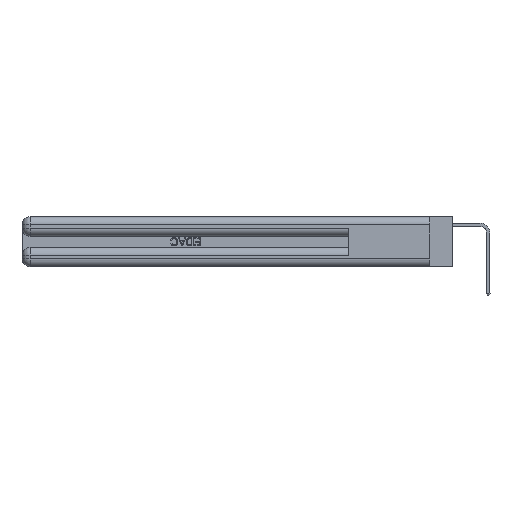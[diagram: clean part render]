
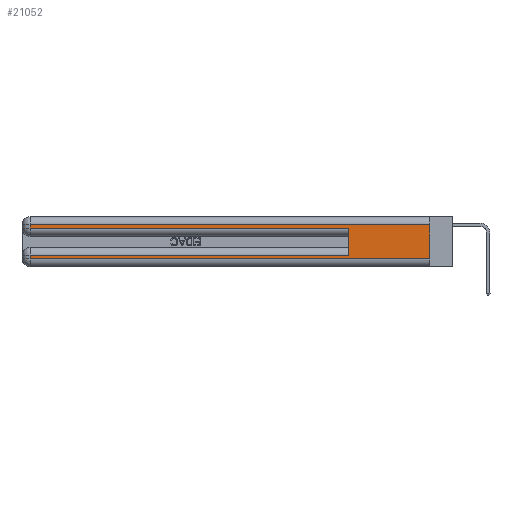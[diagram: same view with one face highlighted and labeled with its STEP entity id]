
A CAD part, left-side view. The second image highlights one B-rep face of the part: STEP entity #21052.
In plain terms, the highlighted planar face has unit normal (-1, 0, 0).
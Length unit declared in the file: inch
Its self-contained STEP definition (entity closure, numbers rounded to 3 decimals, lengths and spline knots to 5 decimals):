
#47 = VECTOR ( 'NONE', #457, 39.37008 ) ;
#259 = DIRECTION ( 'NONE',  ( 0., 1., 0. ) ) ;
#316 = ORIENTED_EDGE ( 'NONE', *, *, #25635, .T. ) ;
#457 = DIRECTION ( 'NONE',  ( 0., 1., 0. ) ) ;
#877 = LINE ( 'NONE', #17049, #5757 ) ;
#927 = AXIS2_PLACEMENT_3D ( 'NONE', #14004, #18781, #24988 ) ;
#1098 = DIRECTION ( 'NONE',  ( 0., 0., -1. ) ) ;
#1578 = FACE_OUTER_BOUND ( 'NONE', #14565, .T. ) ;
#1652 = VERTEX_POINT ( 'NONE', #29674 ) ;
#2261 = CARTESIAN_POINT ( 'NONE',  ( 0., 0., 0.085 ) ) ;
#2672 = VECTOR ( 'NONE', #259, 39.37008 ) ;
#2923 = CARTESIAN_POINT ( 'NONE',  ( 0., 0.6, 0.145 ) ) ;
#3033 = DIRECTION ( 'NONE',  ( 0., -1., 0. ) ) ;
#5238 = LINE ( 'NONE', #2923, #7422 ) ;
#5757 = VECTOR ( 'NONE', #3033, 39.37008 ) ;
#6079 = CARTESIAN_POINT ( 'NONE',  ( 0., 2.94, 0.06 ) ) ;
#6702 = CARTESIAN_POINT ( 'NONE',  ( 0., 2.94, 0.37 ) ) ;
#6934 = ORIENTED_EDGE ( 'NONE', *, *, #9650, .T. ) ;
#7422 = VECTOR ( 'NONE', #26355, 39.37008 ) ;
#7734 = ORIENTED_EDGE ( 'NONE', *, *, #7894, .T. ) ;
#7894 = EDGE_CURVE ( 'NONE', #18151, #29514, #17378, .T. ) ;
#8292 = VECTOR ( 'NONE', #11945, 39.37008 ) ;
#8369 = CARTESIAN_POINT ( 'NONE',  ( 0., 2.94, 0.285 ) ) ;
#9360 = LINE ( 'NONE', #2261, #2672 ) ;
#9480 = LINE ( 'NONE', #6702, #8292 ) ;
#9650 = EDGE_CURVE ( 'NONE', #16815, #29509, #877, .T. ) ;
#10649 = CARTESIAN_POINT ( 'NONE',  ( 0., 2.94, 0.37 ) ) ;
#10735 = CARTESIAN_POINT ( 'NONE',  ( 0., 2.94, 0.085 ) ) ;
#10937 = VECTOR ( 'NONE', #24574, 39.37008 ) ;
#11171 = VECTOR ( 'NONE', #1098, 39.37008 ) ;
#11352 = CARTESIAN_POINT ( 'NONE',  ( 0., 0.6, 0.285 ) ) ;
#11945 = DIRECTION ( 'NONE',  ( 0., 0., -1. ) ) ;
#12612 = CARTESIAN_POINT ( 'NONE',  ( 0., 0., 0.31 ) ) ;
#13238 = ORIENTED_EDGE ( 'NONE', *, *, #16162, .F. ) ;
#13812 = EDGE_CURVE ( 'NONE', #1652, #18993, #9360, .T. ) ;
#14004 = CARTESIAN_POINT ( 'NONE',  ( 0., 0., 0.37 ) ) ;
#14565 = EDGE_LOOP ( 'NONE', ( #13238, #7734, #23786, #28572, #19339, #20364, #316, #6934 ) ) ;
#14960 = LINE ( 'NONE', #10649, #11171 ) ;
#16075 = VECTOR ( 'NONE', #21909, 39.37008 ) ;
#16087 = VERTEX_POINT ( 'NONE', #11352 ) ;
#16162 = EDGE_CURVE ( 'NONE', #18151, #29509, #26422, .T. ) ;
#16466 = PLANE ( 'NONE',  #927 ) ;
#16815 = VERTEX_POINT ( 'NONE', #6079 ) ;
#17049 = CARTESIAN_POINT ( 'NONE',  ( 0., 0., 0.06 ) ) ;
#17378 = LINE ( 'NONE', #12612, #47 ) ;
#17426 = CARTESIAN_POINT ( 'NONE',  ( 0., 2.94, 0.31 ) ) ;
#17476 = VERTEX_POINT ( 'NONE', #8369 ) ;
#18078 = EDGE_CURVE ( 'NONE', #29514, #17476, #14960, .T. ) ;
#18151 = VERTEX_POINT ( 'NONE', #24668 ) ;
#18781 = DIRECTION ( 'NONE',  ( 1., 0., 0. ) ) ;
#18993 = VERTEX_POINT ( 'NONE', #10735 ) ;
#19339 = ORIENTED_EDGE ( 'NONE', *, *, #29838, .F. ) ;
#20364 = ORIENTED_EDGE ( 'NONE', *, *, #13812, .T. ) ;
#21052 = ADVANCED_FACE ( 'NONE', ( #1578 ), #16466, .F. ) ;
#21909 = DIRECTION ( 'NONE',  ( 0., 0., -1. ) ) ;
#21930 = LINE ( 'NONE', #22085, #10937 ) ;
#22085 = CARTESIAN_POINT ( 'NONE',  ( 0., 0., 0.285 ) ) ;
#23046 = EDGE_CURVE ( 'NONE', #17476, #16087, #21930, .T. ) ;
#23786 = ORIENTED_EDGE ( 'NONE', *, *, #18078, .T. ) ;
#24574 = DIRECTION ( 'NONE',  ( 0., -1., 0. ) ) ;
#24668 = CARTESIAN_POINT ( 'NONE',  ( 0., 0., 0.31 ) ) ;
#24988 = DIRECTION ( 'NONE',  ( 0., 0., -1. ) ) ;
#25635 = EDGE_CURVE ( 'NONE', #18993, #16815, #9480, .T. ) ;
#26355 = DIRECTION ( 'NONE',  ( 0., 0., 1. ) ) ;
#26422 = LINE ( 'NONE', #26578, #16075 ) ;
#26578 = CARTESIAN_POINT ( 'NONE',  ( 0., 0., 0.37 ) ) ;
#28572 = ORIENTED_EDGE ( 'NONE', *, *, #23046, .T. ) ;
#29302 = CARTESIAN_POINT ( 'NONE',  ( 0., 0., 0.06 ) ) ;
#29509 = VERTEX_POINT ( 'NONE', #29302 ) ;
#29514 = VERTEX_POINT ( 'NONE', #17426 ) ;
#29674 = CARTESIAN_POINT ( 'NONE',  ( 0., 0.6, 0.085 ) ) ;
#29838 = EDGE_CURVE ( 'NONE', #1652, #16087, #5238, .T. ) ;
